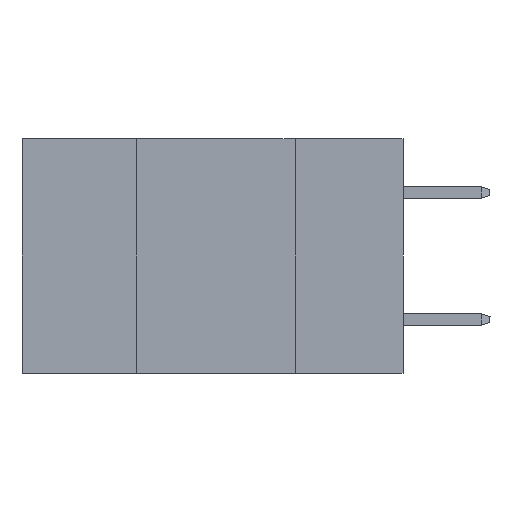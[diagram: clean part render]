
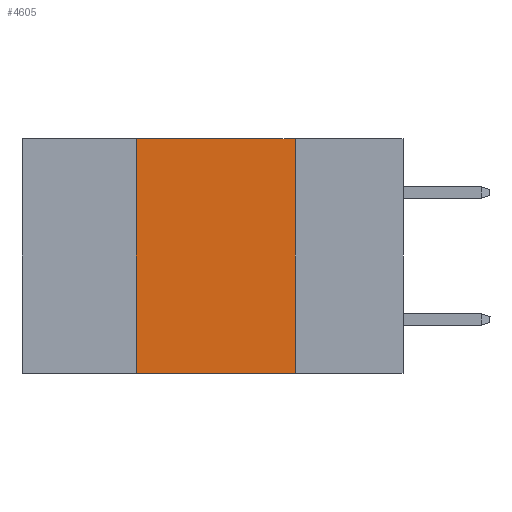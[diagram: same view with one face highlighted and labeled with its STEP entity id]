
A CAD part, left-side view. The second image highlights one B-rep face of the part: STEP entity #4605.
In plain terms, the highlighted planar face has unit normal (-1, 0, 0).
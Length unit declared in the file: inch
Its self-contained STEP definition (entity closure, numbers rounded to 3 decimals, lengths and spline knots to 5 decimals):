
#1230 = VECTOR ( 'NONE', #4206, 39.37008 ) ;
#1605 = VERTEX_POINT ( 'NONE', #24222 ) ;
#1638 = CARTESIAN_POINT ( 'NONE',  ( 0., 0.42, 0. ) ) ;
#1977 = CARTESIAN_POINT ( 'NONE',  ( 0., 0.6, 0. ) ) ;
#3306 = DIRECTION ( 'NONE',  ( 0., -1., 0. ) ) ;
#4206 = DIRECTION ( 'NONE',  ( 0., -1., 0. ) ) ;
#4236 = ORIENTED_EDGE ( 'NONE', *, *, #11490, .F. ) ;
#4605 = ADVANCED_FACE ( 'NONE', ( #14996 ), #19238, .F. ) ;
#4889 = EDGE_CURVE ( 'NONE', #15287, #5463, #10551, .T. ) ;
#5463 = VERTEX_POINT ( 'NONE', #20611 ) ;
#5747 = DIRECTION ( 'NONE',  ( 0., 0., 1. ) ) ;
#6783 = EDGE_LOOP ( 'NONE', ( #17926, #20831, #4236, #8170 ) ) ;
#7302 = LINE ( 'NONE', #24038, #19233 ) ;
#8170 = ORIENTED_EDGE ( 'NONE', *, *, #15299, .T. ) ;
#10551 = LINE ( 'NONE', #1977, #1230 ) ;
#11002 = CARTESIAN_POINT ( 'NONE',  ( 0., 0.17, 0. ) ) ;
#11490 = EDGE_CURVE ( 'NONE', #1605, #15287, #7302, .T. ) ;
#12329 = VERTEX_POINT ( 'NONE', #25846 ) ;
#12670 = VECTOR ( 'NONE', #21425, 39.37008 ) ;
#14996 = FACE_OUTER_BOUND ( 'NONE', #6783, .T. ) ;
#15287 = VERTEX_POINT ( 'NONE', #1638 ) ;
#15299 = EDGE_CURVE ( 'NONE', #1605, #12329, #26744, .T. ) ;
#15882 = CARTESIAN_POINT ( 'NONE',  ( 0., 0.6, -0.37 ) ) ;
#17926 = ORIENTED_EDGE ( 'NONE', *, *, #26557, .F. ) ;
#18879 = VECTOR ( 'NONE', #3306, 39.37008 ) ;
#19233 = VECTOR ( 'NONE', #5747, 39.37008 ) ;
#19238 = PLANE ( 'NONE',  #25402 ) ;
#19781 = DIRECTION ( 'NONE',  ( 0., 0., -1. ) ) ;
#20611 = CARTESIAN_POINT ( 'NONE',  ( 0., 0.17, 0. ) ) ;
#20831 = ORIENTED_EDGE ( 'NONE', *, *, #4889, .F. ) ;
#21425 = DIRECTION ( 'NONE',  ( 0., 0., -1. ) ) ;
#24038 = CARTESIAN_POINT ( 'NONE',  ( 0., 0.42, 0. ) ) ;
#24061 = DIRECTION ( 'NONE',  ( 1., 0., 0. ) ) ;
#24222 = CARTESIAN_POINT ( 'NONE',  ( 0., 0.42, -0.37 ) ) ;
#25144 = LINE ( 'NONE', #11002, #12670 ) ;
#25402 = AXIS2_PLACEMENT_3D ( 'NONE', #26258, #24061, #19781 ) ;
#25846 = CARTESIAN_POINT ( 'NONE',  ( 0., 0.17, -0.37 ) ) ;
#26258 = CARTESIAN_POINT ( 'NONE',  ( 0., 0.6, 0. ) ) ;
#26557 = EDGE_CURVE ( 'NONE', #5463, #12329, #25144, .T. ) ;
#26744 = LINE ( 'NONE', #15882, #18879 ) ;
